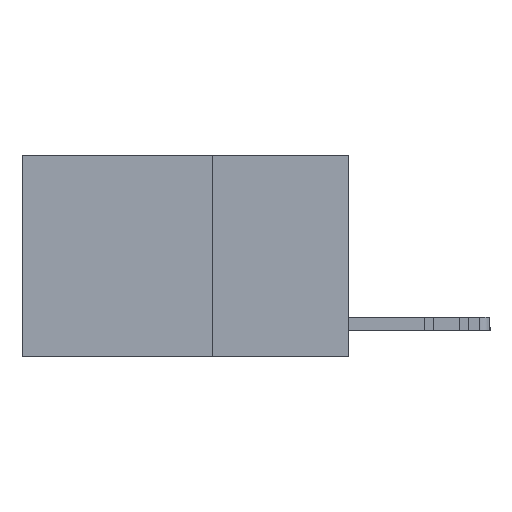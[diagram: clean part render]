
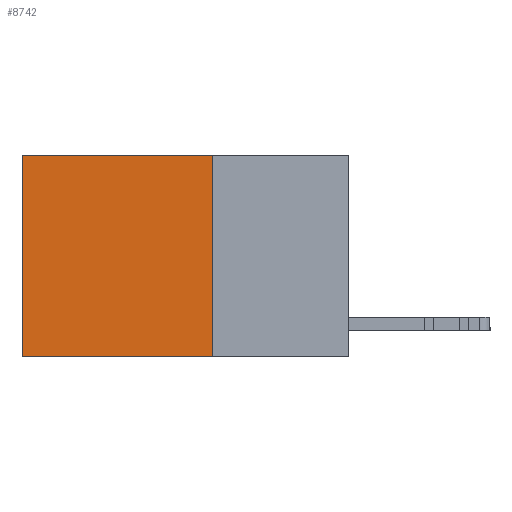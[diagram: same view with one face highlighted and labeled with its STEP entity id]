
A CAD part, left-side view. The second image highlights one B-rep face of the part: STEP entity #8742.
In plain terms, the highlighted planar face has unit normal (-1, 0, 0).
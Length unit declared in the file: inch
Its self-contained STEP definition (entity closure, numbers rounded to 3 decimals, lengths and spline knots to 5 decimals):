
#708 = AXIS2_PLACEMENT_3D ( 'NONE', #3510, #11971, #16573 ) ;
#1988 = FACE_OUTER_BOUND ( 'NONE', #20024, .T. ) ;
#2380 = CARTESIAN_POINT ( 'NONE',  ( 0.2625, 0.6, -0.37 ) ) ;
#2694 = LINE ( 'NONE', #19590, #3535 ) ;
#2711 = CARTESIAN_POINT ( 'NONE',  ( 0.2625, 0.25, -0.37 ) ) ;
#2997 = ORIENTED_EDGE ( 'NONE', *, *, #15783, .T. ) ;
#3260 = CARTESIAN_POINT ( 'NONE',  ( 0.2625, 0.6, 0. ) ) ;
#3510 = CARTESIAN_POINT ( 'NONE',  ( 0.2625, 0.25, 0. ) ) ;
#3535 = VECTOR ( 'NONE', #11552, 39.37008 ) ;
#4503 = ORIENTED_EDGE ( 'NONE', *, *, #11868, .T. ) ;
#4988 = DIRECTION ( 'NONE',  ( 0., 0., -1. ) ) ;
#6626 = DIRECTION ( 'NONE',  ( 0., 1., 0. ) ) ;
#6634 = CARTESIAN_POINT ( 'NONE',  ( 0.2625, 0.6, 0. ) ) ;
#6855 = VERTEX_POINT ( 'NONE', #3260 ) ;
#7568 = DIRECTION ( 'NONE',  ( 0., 0., -1. ) ) ;
#8742 = ADVANCED_FACE ( 'NONE', ( #1988 ), #16301, .F. ) ;
#9803 = VERTEX_POINT ( 'NONE', #2711 ) ;
#11552 = DIRECTION ( 'NONE',  ( 0., 1., 0. ) ) ;
#11868 = EDGE_CURVE ( 'NONE', #6855, #18864, #13040, .T. ) ;
#11971 = DIRECTION ( 'NONE',  ( 1., 0., 0. ) ) ;
#12193 = LINE ( 'NONE', #20486, #24804 ) ;
#13040 = LINE ( 'NONE', #6634, #14727 ) ;
#14727 = VECTOR ( 'NONE', #4988, 39.37008 ) ;
#15783 = EDGE_CURVE ( 'NONE', #18933, #6855, #2694, .T. ) ;
#16301 = PLANE ( 'NONE',  #708 ) ;
#16573 = DIRECTION ( 'NONE',  ( 0., 0., -1. ) ) ;
#17369 = EDGE_CURVE ( 'NONE', #9803, #18864, #23100, .T. ) ;
#18864 = VERTEX_POINT ( 'NONE', #2380 ) ;
#18933 = VERTEX_POINT ( 'NONE', #22819 ) ;
#19458 = EDGE_CURVE ( 'NONE', #18933, #9803, #12193, .T. ) ;
#19590 = CARTESIAN_POINT ( 'NONE',  ( 0.2625, 0.25, 0. ) ) ;
#20024 = EDGE_LOOP ( 'NONE', ( #4503, #22236, #24176, #2997 ) ) ;
#20486 = CARTESIAN_POINT ( 'NONE',  ( 0.2625, 0.25, 0. ) ) ;
#22236 = ORIENTED_EDGE ( 'NONE', *, *, #17369, .F. ) ;
#22819 = CARTESIAN_POINT ( 'NONE',  ( 0.2625, 0.25, 0. ) ) ;
#23100 = LINE ( 'NONE', #25299, #26475 ) ;
#24176 = ORIENTED_EDGE ( 'NONE', *, *, #19458, .F. ) ;
#24804 = VECTOR ( 'NONE', #7568, 39.37008 ) ;
#25299 = CARTESIAN_POINT ( 'NONE',  ( 0.2625, 0.25, -0.37 ) ) ;
#26475 = VECTOR ( 'NONE', #6626, 39.37008 ) ;
